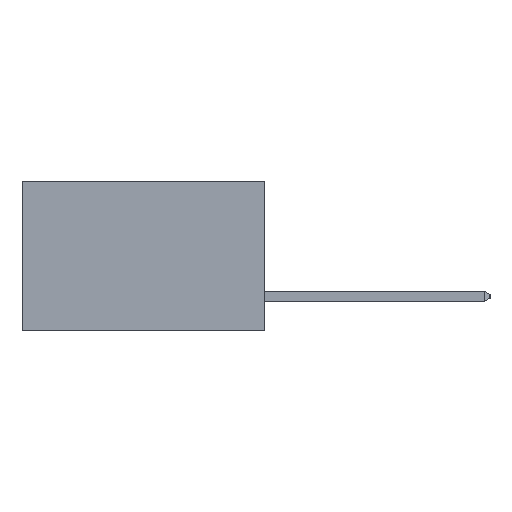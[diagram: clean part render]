
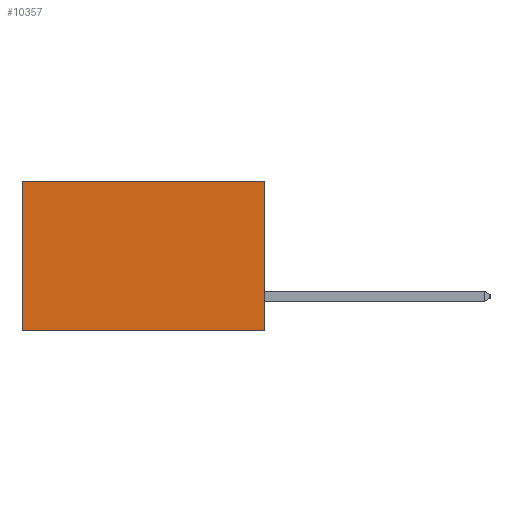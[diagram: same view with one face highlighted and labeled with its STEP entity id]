
A CAD part, left-side view. The second image highlights one B-rep face of the part: STEP entity #10357.
In plain terms, the highlighted planar face has unit normal (-1, 0, 0).
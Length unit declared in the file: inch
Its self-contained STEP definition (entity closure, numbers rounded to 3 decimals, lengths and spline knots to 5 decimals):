
#6 = VERTEX_POINT ( 'NONE', #2322 ) ;
#264 = VERTEX_POINT ( 'NONE', #11344 ) ;
#393 = CARTESIAN_POINT ( 'NONE',  ( 0.2615, 0., -0.37 ) ) ;
#428 = VERTEX_POINT ( 'NONE', #4128 ) ;
#1532 = LINE ( 'NONE', #12798, #9902 ) ;
#1578 = DIRECTION ( 'NONE',  ( 0., 0., -1. ) ) ;
#2271 = PLANE ( 'NONE',  #3982 ) ;
#2322 = CARTESIAN_POINT ( 'NONE',  ( 0.2615, 0., 0. ) ) ;
#2417 = LINE ( 'NONE', #10589, #12325 ) ;
#2890 = LINE ( 'NONE', #393, #11140 ) ;
#3385 = EDGE_CURVE ( 'NONE', #428, #264, #12314, .T. ) ;
#3982 = AXIS2_PLACEMENT_3D ( 'NONE', #10326, #4299, #11265 ) ;
#4128 = CARTESIAN_POINT ( 'NONE',  ( 0.2615, 0.6, 0. ) ) ;
#4299 = DIRECTION ( 'NONE',  ( 1., 0., 0. ) ) ;
#4655 = ORIENTED_EDGE ( 'NONE', *, *, #3385, .T. ) ;
#5260 = EDGE_LOOP ( 'NONE', ( #4655, #10955, #6555, #11477 ) ) ;
#5700 = EDGE_CURVE ( 'NONE', #6, #428, #1532, .T. ) ;
#5745 = VERTEX_POINT ( 'NONE', #12129 ) ;
#6555 = ORIENTED_EDGE ( 'NONE', *, *, #11730, .F. ) ;
#7517 = DIRECTION ( 'NONE',  ( 0., 1., 0. ) ) ;
#9076 = FACE_OUTER_BOUND ( 'NONE', #5260, .T. ) ;
#9511 = DIRECTION ( 'NONE',  ( 0., 0., -1. ) ) ;
#9516 = VECTOR ( 'NONE', #9511, 39.37008 ) ;
#9559 = CARTESIAN_POINT ( 'NONE',  ( 0.2615, 0.6, -0.37 ) ) ;
#9902 = VECTOR ( 'NONE', #12472, 39.37008 ) ;
#10326 = CARTESIAN_POINT ( 'NONE',  ( 0.2615, 0., -0.37 ) ) ;
#10357 = ADVANCED_FACE ( 'NONE', ( #9076 ), #2271, .F. ) ;
#10589 = CARTESIAN_POINT ( 'NONE',  ( 0.2615, 0., -0.37 ) ) ;
#10955 = ORIENTED_EDGE ( 'NONE', *, *, #12301, .F. ) ;
#11140 = VECTOR ( 'NONE', #7517, 39.37008 ) ;
#11265 = DIRECTION ( 'NONE',  ( 0., 0., -1. ) ) ;
#11344 = CARTESIAN_POINT ( 'NONE',  ( 0.2615, 0.6, -0.37 ) ) ;
#11477 = ORIENTED_EDGE ( 'NONE', *, *, #5700, .T. ) ;
#11730 = EDGE_CURVE ( 'NONE', #6, #5745, #2417, .T. ) ;
#12129 = CARTESIAN_POINT ( 'NONE',  ( 0.2615, 0., -0.37 ) ) ;
#12301 = EDGE_CURVE ( 'NONE', #5745, #264, #2890, .T. ) ;
#12314 = LINE ( 'NONE', #9559, #9516 ) ;
#12325 = VECTOR ( 'NONE', #1578, 39.37008 ) ;
#12472 = DIRECTION ( 'NONE',  ( 0., 1., 0. ) ) ;
#12798 = CARTESIAN_POINT ( 'NONE',  ( 0.2615, 0., 0. ) ) ;
